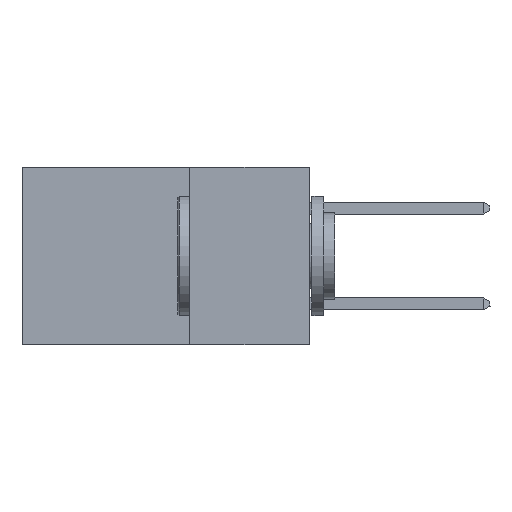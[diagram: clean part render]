
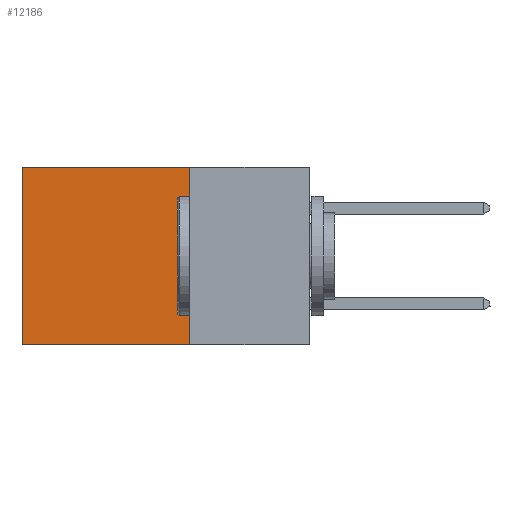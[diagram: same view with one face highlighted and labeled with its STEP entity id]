
A CAD part, left-side view. The second image highlights one B-rep face of the part: STEP entity #12186.
In plain terms, the highlighted planar face has unit normal (-1, 0, 0).
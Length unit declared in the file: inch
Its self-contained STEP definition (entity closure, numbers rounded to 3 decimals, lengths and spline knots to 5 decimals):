
#43 = AXIS2_PLACEMENT_3D ( 'NONE', #11861, #24072, #11945 ) ;
#3042 = EDGE_LOOP ( 'NONE', ( #7220, #6031, #7950, #20729 ) ) ;
#3072 = VERTEX_POINT ( 'NONE', #8913 ) ;
#3143 = CARTESIAN_POINT ( 'NONE',  ( 0.2875, 0.25, 0. ) ) ;
#4691 = EDGE_CURVE ( 'NONE', #22555, #20752, #21469, .T. ) ;
#5332 = VECTOR ( 'NONE', #25177, 39.37008 ) ;
#6031 = ORIENTED_EDGE ( 'NONE', *, *, #4691, .F. ) ;
#6171 = VECTOR ( 'NONE', #11693, 39.37008 ) ;
#6237 = CARTESIAN_POINT ( 'NONE',  ( 0.2875, 0.25, -0.37 ) ) ;
#7220 = ORIENTED_EDGE ( 'NONE', *, *, #16227, .T. ) ;
#7352 = DIRECTION ( 'NONE',  ( 0., 1., 0. ) ) ;
#7512 = VECTOR ( 'NONE', #7352, 39.37008 ) ;
#7950 = ORIENTED_EDGE ( 'NONE', *, *, #19457, .F. ) ;
#8913 = CARTESIAN_POINT ( 'NONE',  ( 0.2875, 0.6, 0. ) ) ;
#9642 = CARTESIAN_POINT ( 'NONE',  ( 0.2875, 0.6, 0. ) ) ;
#9646 = DIRECTION ( 'NONE',  ( 0., 1., 0. ) ) ;
#10621 = VECTOR ( 'NONE', #9646, 39.37008 ) ;
#11048 = CARTESIAN_POINT ( 'NONE',  ( 0.2875, 0.25, 0. ) ) ;
#11287 = FACE_OUTER_BOUND ( 'NONE', #3042, .T. ) ;
#11447 = EDGE_CURVE ( 'NONE', #13190, #3072, #12300, .T. ) ;
#11693 = DIRECTION ( 'NONE',  ( 0., 0., -1. ) ) ;
#11861 = CARTESIAN_POINT ( 'NONE',  ( 0.2875, 0.25, 0. ) ) ;
#11945 = DIRECTION ( 'NONE',  ( 0., 0., -1. ) ) ;
#12186 = ADVANCED_FACE ( 'NONE', ( #11287 ), #22094, .F. ) ;
#12300 = LINE ( 'NONE', #3143, #7512 ) ;
#13190 = VERTEX_POINT ( 'NONE', #25323 ) ;
#13683 = CARTESIAN_POINT ( 'NONE',  ( 0.2875, 0.25, -0.37 ) ) ;
#16227 = EDGE_CURVE ( 'NONE', #3072, #20752, #22433, .T. ) ;
#16745 = CARTESIAN_POINT ( 'NONE',  ( 0.2875, 0.6, -0.37 ) ) ;
#16844 = LINE ( 'NONE', #11048, #5332 ) ;
#19457 = EDGE_CURVE ( 'NONE', #13190, #22555, #16844, .T. ) ;
#20729 = ORIENTED_EDGE ( 'NONE', *, *, #11447, .T. ) ;
#20752 = VERTEX_POINT ( 'NONE', #16745 ) ;
#21469 = LINE ( 'NONE', #13683, #10621 ) ;
#22094 = PLANE ( 'NONE',  #43 ) ;
#22433 = LINE ( 'NONE', #9642, #6171 ) ;
#22555 = VERTEX_POINT ( 'NONE', #6237 ) ;
#24072 = DIRECTION ( 'NONE',  ( 1., 0., 0. ) ) ;
#25177 = DIRECTION ( 'NONE',  ( 0., 0., -1. ) ) ;
#25323 = CARTESIAN_POINT ( 'NONE',  ( 0.2875, 0.25, 0. ) ) ;
